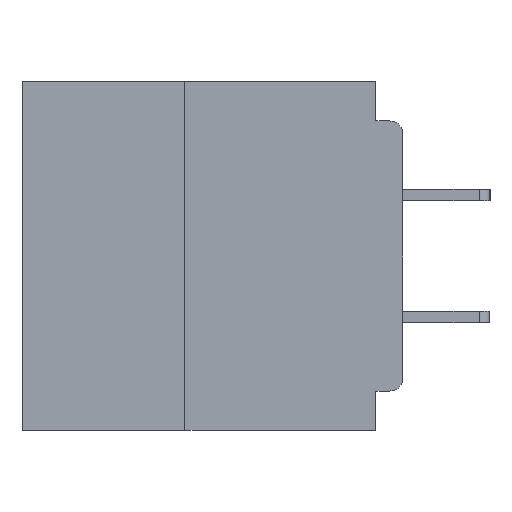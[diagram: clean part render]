
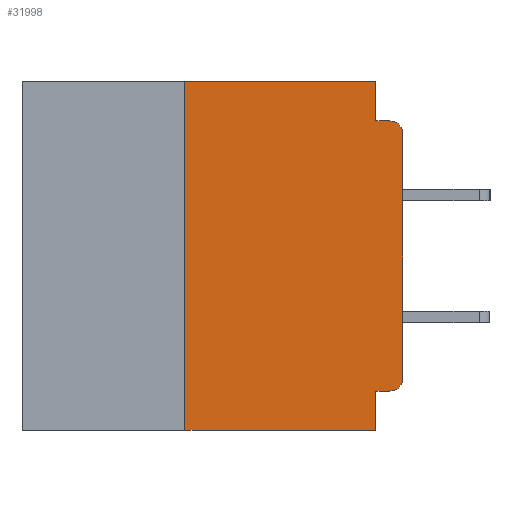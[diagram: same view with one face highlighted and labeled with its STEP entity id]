
A CAD part, left-side view. The second image highlights one B-rep face of the part: STEP entity #31998.
In plain terms, the highlighted planar face has unit normal (-1, 0, 0).
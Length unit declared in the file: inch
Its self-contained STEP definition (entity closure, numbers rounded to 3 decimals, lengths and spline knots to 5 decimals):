
#367 = ORIENTED_EDGE ( 'NONE', *, *, #47399, .F. ) ;
#810 = ORIENTED_EDGE ( 'NONE', *, *, #58068, .F. ) ;
#834 = DIRECTION ( 'NONE',  ( -1., 0., 0. ) ) ;
#1021 = PLANE ( 'NONE',  #55144 ) ;
#1636 = LINE ( 'NONE', #24535, #43405 ) ;
#2338 = CARTESIAN_POINT ( 'NONE',  ( 0., 0.031, -0.4 ) ) ;
#3157 = CARTESIAN_POINT ( 'NONE',  ( 0., 0.031, -0.355 ) ) ;
#3516 = ORIENTED_EDGE ( 'NONE', *, *, #22579, .F. ) ;
#3573 = VERTEX_POINT ( 'NONE', #41913 ) ;
#3767 = ORIENTED_EDGE ( 'NONE', *, *, #31528, .F. ) ;
#6140 = DIRECTION ( 'NONE',  ( 0., 0., -1. ) ) ;
#6555 = VECTOR ( 'NONE', #62399, 39.37008 ) ;
#6993 = VECTOR ( 'NONE', #49699, 39.37008 ) ;
#7367 = CARTESIAN_POINT ( 'NONE',  ( 0., 0.25, -0.4 ) ) ;
#7729 = CARTESIAN_POINT ( 'NONE',  ( 0., 0.015, -0.355 ) ) ;
#10680 = CIRCLE ( 'NONE', #21223, 0.015 ) ;
#12037 = ORIENTED_EDGE ( 'NONE', *, *, #46945, .T. ) ;
#12933 = VERTEX_POINT ( 'NONE', #7367 ) ;
#14227 = FACE_OUTER_BOUND ( 'NONE', #50665, .T. ) ;
#14603 = ORIENTED_EDGE ( 'NONE', *, *, #40296, .F. ) ;
#16086 = VERTEX_POINT ( 'NONE', #29733 ) ;
#16575 = CARTESIAN_POINT ( 'NONE',  ( 0., 0., -0.355 ) ) ;
#17809 = LINE ( 'NONE', #46415, #29635 ) ;
#19124 = CARTESIAN_POINT ( 'NONE',  ( 0., 0.031, 0. ) ) ;
#21223 = AXIS2_PLACEMENT_3D ( 'NONE', #31129, #834, #36192 ) ;
#21308 = CARTESIAN_POINT ( 'NONE',  ( 0., 0.015, -0.045 ) ) ;
#21392 = CARTESIAN_POINT ( 'NONE',  ( 0., 0.015, -0.34 ) ) ;
#21505 = DIRECTION ( 'NONE',  ( 0., 0., 1. ) ) ;
#21886 = EDGE_CURVE ( 'NONE', #12933, #16086, #17809, .T. ) ;
#22320 = VERTEX_POINT ( 'NONE', #60980 ) ;
#22334 = CARTESIAN_POINT ( 'NONE',  ( 0., 0., 0. ) ) ;
#22579 = EDGE_CURVE ( 'NONE', #32563, #3573, #31225, .T. ) ;
#23155 = VERTEX_POINT ( 'NONE', #3157 ) ;
#24255 = ORIENTED_EDGE ( 'NONE', *, *, #21886, .F. ) ;
#24535 = CARTESIAN_POINT ( 'NONE',  ( 0., 0.031, -0.4 ) ) ;
#24563 = VECTOR ( 'NONE', #41633, 39.37008 ) ;
#24882 = CARTESIAN_POINT ( 'NONE',  ( 0., 0., -0.045 ) ) ;
#25854 = LINE ( 'NONE', #22334, #37665 ) ;
#26459 = DIRECTION ( 'NONE',  ( 0., 0., -1. ) ) ;
#27400 = DIRECTION ( 'NONE',  ( 0., 0., 1. ) ) ;
#28786 = ORIENTED_EDGE ( 'NONE', *, *, #55548, .T. ) ;
#29201 = ORIENTED_EDGE ( 'NONE', *, *, #35606, .T. ) ;
#29635 = VECTOR ( 'NONE', #21505, 39.37008 ) ;
#29733 = CARTESIAN_POINT ( 'NONE',  ( 0., 0.25, 0. ) ) ;
#31129 = CARTESIAN_POINT ( 'NONE',  ( 0., 0.015, -0.06 ) ) ;
#31225 = LINE ( 'NONE', #19124, #57630 ) ;
#31528 = EDGE_CURVE ( 'NONE', #35826, #23155, #39502, .T. ) ;
#31827 = ORIENTED_EDGE ( 'NONE', *, *, #33527, .T. ) ;
#31998 = ADVANCED_FACE ( 'NONE', ( #14227 ), #1021, .F. ) ;
#32563 = VERTEX_POINT ( 'NONE', #35216 ) ;
#32671 = VERTEX_POINT ( 'NONE', #21308 ) ;
#33527 = EDGE_CURVE ( 'NONE', #63581, #22320, #25854, .T. ) ;
#33839 = LINE ( 'NONE', #24882, #6993 ) ;
#35216 = CARTESIAN_POINT ( 'NONE',  ( 0., 0.031, 0. ) ) ;
#35606 = EDGE_CURVE ( 'NONE', #12933, #47112, #45070, .T. ) ;
#35826 = VERTEX_POINT ( 'NONE', #7729 ) ;
#36166 = DIRECTION ( 'NONE',  ( 1., 0., 0. ) ) ;
#36192 = DIRECTION ( 'NONE',  ( 0., 0., -1. ) ) ;
#37665 = VECTOR ( 'NONE', #27400, 39.37008 ) ;
#38623 = AXIS2_PLACEMENT_3D ( 'NONE', #21392, #56238, #26459 ) ;
#39502 = LINE ( 'NONE', #16575, #24563 ) ;
#40296 = EDGE_CURVE ( 'NONE', #16086, #32563, #46585, .T. ) ;
#41215 = CARTESIAN_POINT ( 'NONE',  ( 0., 0.437, -0.4 ) ) ;
#41633 = DIRECTION ( 'NONE',  ( 0., 1., 0. ) ) ;
#41913 = CARTESIAN_POINT ( 'NONE',  ( 0., 0.031, -0.045 ) ) ;
#43405 = VECTOR ( 'NONE', #59327, 39.37008 ) ;
#45070 = LINE ( 'NONE', #41215, #56672 ) ;
#46415 = CARTESIAN_POINT ( 'NONE',  ( 0., 0.25, -0.4 ) ) ;
#46585 = LINE ( 'NONE', #47443, #6555 ) ;
#46945 = EDGE_CURVE ( 'NONE', #35826, #63581, #61809, .T. ) ;
#47112 = VERTEX_POINT ( 'NONE', #2338 ) ;
#47399 = EDGE_CURVE ( 'NONE', #3573, #32671, #33839, .T. ) ;
#47443 = CARTESIAN_POINT ( 'NONE',  ( 0., 0.437, 0. ) ) ;
#49261 = CARTESIAN_POINT ( 'NONE',  ( 0., 0., -0.34 ) ) ;
#49699 = DIRECTION ( 'NONE',  ( 0., -1., 0. ) ) ;
#50665 = EDGE_LOOP ( 'NONE', ( #31827, #28786, #367, #3516, #14603, #24255, #29201, #810, #3767, #12037 ) ) ;
#54047 = DIRECTION ( 'NONE',  ( 0., 0., -1. ) ) ;
#55144 = AXIS2_PLACEMENT_3D ( 'NONE', #61022, #36166, #6140 ) ;
#55548 = EDGE_CURVE ( 'NONE', #22320, #32671, #10680, .T. ) ;
#56238 = DIRECTION ( 'NONE',  ( -1., 0., 0. ) ) ;
#56672 = VECTOR ( 'NONE', #60847, 39.37008 ) ;
#57630 = VECTOR ( 'NONE', #54047, 39.37008 ) ;
#58068 = EDGE_CURVE ( 'NONE', #23155, #47112, #1636, .T. ) ;
#59327 = DIRECTION ( 'NONE',  ( 0., 0., -1. ) ) ;
#60847 = DIRECTION ( 'NONE',  ( 0., -1., 0. ) ) ;
#60980 = CARTESIAN_POINT ( 'NONE',  ( 0., 0., -0.06 ) ) ;
#61022 = CARTESIAN_POINT ( 'NONE',  ( 0., 0.437, 0. ) ) ;
#61809 = CIRCLE ( 'NONE', #38623, 0.015 ) ;
#62399 = DIRECTION ( 'NONE',  ( 0., -1., 0. ) ) ;
#63581 = VERTEX_POINT ( 'NONE', #49261 ) ;
